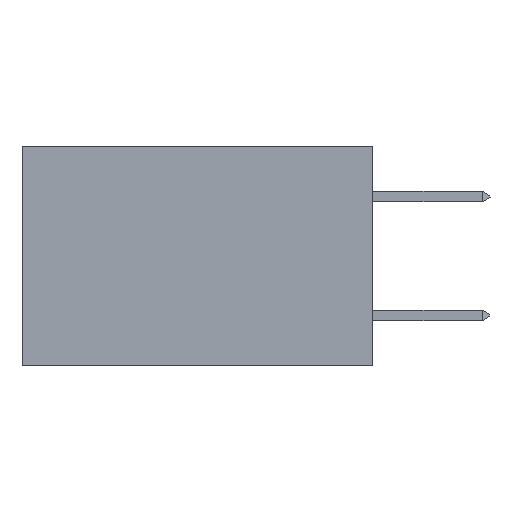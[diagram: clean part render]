
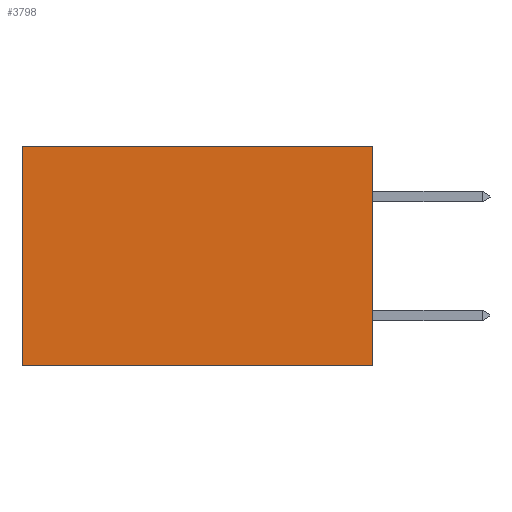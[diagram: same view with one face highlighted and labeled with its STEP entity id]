
A CAD part, left-side view. The second image highlights one B-rep face of the part: STEP entity #3798.
In plain terms, the highlighted planar face has unit normal (-1, 0, 0).
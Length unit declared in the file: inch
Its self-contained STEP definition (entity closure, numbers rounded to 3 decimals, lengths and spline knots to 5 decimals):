
#770 = VERTEX_POINT ( 'NONE', #1556 ) ;
#1078 = VECTOR ( 'NONE', #3088, 39.37008 ) ;
#1446 = PLANE ( 'NONE',  #10164 ) ;
#1556 = CARTESIAN_POINT ( 'NONE',  ( 0.277, 0., 0. ) ) ;
#2519 = DIRECTION ( 'NONE',  ( 0., 0., -1. ) ) ;
#2738 = VERTEX_POINT ( 'NONE', #5852 ) ;
#3085 = VERTEX_POINT ( 'NONE', #9391 ) ;
#3088 = DIRECTION ( 'NONE',  ( 0., 1., 0. ) ) ;
#3093 = VECTOR ( 'NONE', #2519, 39.37008 ) ;
#3100 = EDGE_CURVE ( 'NONE', #3085, #7547, #10333, .T. ) ;
#3325 = EDGE_CURVE ( 'NONE', #770, #3085, #10709, .T. ) ;
#3663 = EDGE_CURVE ( 'NONE', #770, #2738, #7853, .T. ) ;
#3798 = ADVANCED_FACE ( 'NONE', ( #9308 ), #1446, .F. ) ;
#4150 = DIRECTION ( 'NONE',  ( 0., 0., -1. ) ) ;
#4581 = ORIENTED_EDGE ( 'NONE', *, *, #10244, .T. ) ;
#4592 = ORIENTED_EDGE ( 'NONE', *, *, #3100, .F. ) ;
#4831 = ORIENTED_EDGE ( 'NONE', *, *, #3325, .F. ) ;
#4841 = ORIENTED_EDGE ( 'NONE', *, *, #3663, .T. ) ;
#5136 = CARTESIAN_POINT ( 'NONE',  ( 0.277, 0.59, -0.37 ) ) ;
#5547 = DIRECTION ( 'NONE',  ( 0., 1., 0. ) ) ;
#5597 = EDGE_LOOP ( 'NONE', ( #4581, #4592, #4831, #4841 ) ) ;
#5852 = CARTESIAN_POINT ( 'NONE',  ( 0.277, 0.59, 0. ) ) ;
#5947 = CARTESIAN_POINT ( 'NONE',  ( 0.277, 0., -0.37 ) ) ;
#7547 = VERTEX_POINT ( 'NONE', #10240 ) ;
#7597 = CARTESIAN_POINT ( 'NONE',  ( 0.277, 0., -0.37 ) ) ;
#7707 = LINE ( 'NONE', #5136, #3093 ) ;
#7853 = LINE ( 'NONE', #8276, #1078 ) ;
#8270 = VECTOR ( 'NONE', #11136, 39.37008 ) ;
#8276 = CARTESIAN_POINT ( 'NONE',  ( 0.277, 0., 0. ) ) ;
#9299 = DIRECTION ( 'NONE',  ( 1., 0., 0. ) ) ;
#9308 = FACE_OUTER_BOUND ( 'NONE', #5597, .T. ) ;
#9391 = CARTESIAN_POINT ( 'NONE',  ( 0.277, 0., -0.37 ) ) ;
#10164 = AXIS2_PLACEMENT_3D ( 'NONE', #7597, #9299, #4150 ) ;
#10240 = CARTESIAN_POINT ( 'NONE',  ( 0.277, 0.59, -0.37 ) ) ;
#10244 = EDGE_CURVE ( 'NONE', #2738, #7547, #7707, .T. ) ;
#10333 = LINE ( 'NONE', #5947, #10582 ) ;
#10582 = VECTOR ( 'NONE', #5547, 39.37008 ) ;
#10709 = LINE ( 'NONE', #11213, #8270 ) ;
#11136 = DIRECTION ( 'NONE',  ( 0., 0., -1. ) ) ;
#11213 = CARTESIAN_POINT ( 'NONE',  ( 0.277, 0., -0.37 ) ) ;
